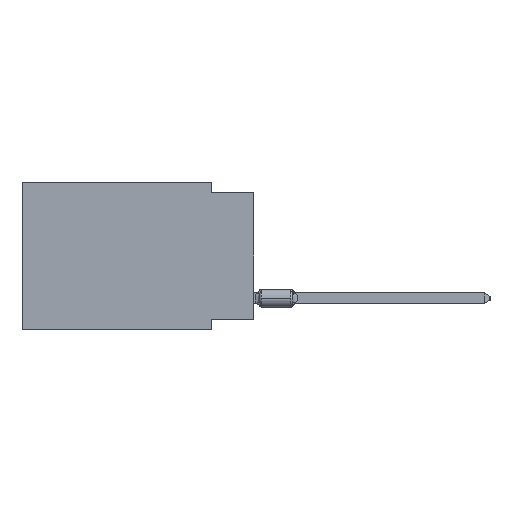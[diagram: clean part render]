
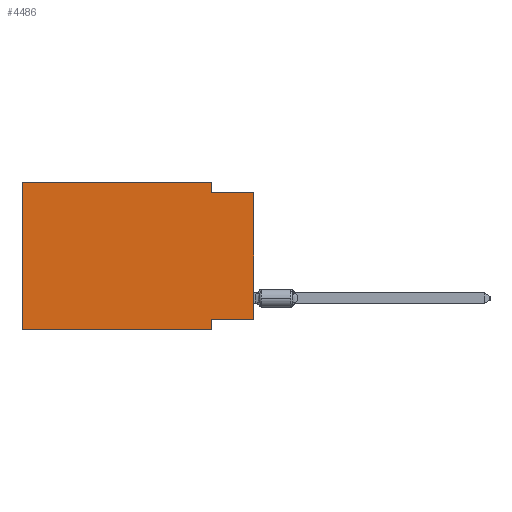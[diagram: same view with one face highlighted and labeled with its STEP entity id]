
A CAD part, left-side view. The second image highlights one B-rep face of the part: STEP entity #4486.
In plain terms, the highlighted planar face has unit normal (-1, 0, 0).
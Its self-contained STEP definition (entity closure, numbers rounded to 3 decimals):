
#250 = CARTESIAN_POINT ( 'NONE',  ( 0., 13.97, -8.89 ) ) ;
#287 = VERTEX_POINT ( 'NONE', #46574 ) ;
#1240 = EDGE_CURVE ( 'NONE', #6815, #39775, #16310, .T. ) ;
#1781 = EDGE_CURVE ( 'NONE', #7758, #39775, #43823, .T. ) ;
#1793 = EDGE_CURVE ( 'NONE', #24050, #10209, #14880, .T. ) ;
#2637 = VECTOR ( 'NONE', #41214, 1000. ) ;
#2808 = VERTEX_POINT ( 'NONE', #15003 ) ;
#3193 = DIRECTION ( 'NONE',  ( 0., 0., 1. ) ) ;
#3563 = CARTESIAN_POINT ( 'NONE',  ( 0., 2.54, -8.89 ) ) ;
#4158 = DIRECTION ( 'NONE',  ( 0., -1., 0. ) ) ;
#4486 = ADVANCED_FACE ( 'NONE', ( #8408 ), #12046, .F. ) ;
#5541 = AXIS2_PLACEMENT_3D ( 'NONE', #26904, #27388, #34438 ) ;
#5561 = CARTESIAN_POINT ( 'NONE',  ( 0., 13.97, -8.89 ) ) ;
#6062 = ORIENTED_EDGE ( 'NONE', *, *, #19565, .F. ) ;
#6815 = VERTEX_POINT ( 'NONE', #19381 ) ;
#7599 = LINE ( 'NONE', #34134, #39858 ) ;
#7758 = VERTEX_POINT ( 'NONE', #9679 ) ;
#7832 = VERTEX_POINT ( 'NONE', #5561 ) ;
#8134 = VECTOR ( 'NONE', #27026, 1000. ) ;
#8164 = CARTESIAN_POINT ( 'NONE',  ( 0., 2.54, 0. ) ) ;
#8408 = FACE_OUTER_BOUND ( 'NONE', #32817, .T. ) ;
#9679 = CARTESIAN_POINT ( 'NONE',  ( 0., 0., -8.255 ) ) ;
#10209 = VERTEX_POINT ( 'NONE', #8164 ) ;
#11531 = CARTESIAN_POINT ( 'NONE',  ( 0., 13.97, 0. ) ) ;
#11542 = CARTESIAN_POINT ( 'NONE',  ( 0., 13.97, 0. ) ) ;
#12046 = PLANE ( 'NONE',  #5541 ) ;
#12173 = CARTESIAN_POINT ( 'NONE',  ( 0., 0., -0.635 ) ) ;
#12879 = EDGE_CURVE ( 'NONE', #10209, #6815, #7599, .T. ) ;
#13235 = VECTOR ( 'NONE', #3193, 1000. ) ;
#13362 = EDGE_CURVE ( 'NONE', #7832, #2808, #33108, .T. ) ;
#14880 = LINE ( 'NONE', #41148, #31129 ) ;
#15003 = CARTESIAN_POINT ( 'NONE',  ( 0., 2.54, -8.89 ) ) ;
#15240 = LINE ( 'NONE', #23019, #30817 ) ;
#16310 = LINE ( 'NONE', #12173, #8134 ) ;
#16753 = ORIENTED_EDGE ( 'NONE', *, *, #1240, .F. ) ;
#18313 = DIRECTION ( 'NONE',  ( 0., 0., -1. ) ) ;
#18739 = ORIENTED_EDGE ( 'NONE', *, *, #13362, .T. ) ;
#19381 = CARTESIAN_POINT ( 'NONE',  ( 0., 2.54, -0.635 ) ) ;
#19565 = EDGE_CURVE ( 'NONE', #7758, #287, #15240, .T. ) ;
#22306 = DIRECTION ( 'NONE',  ( 0., 0., -1. ) ) ;
#22480 = LINE ( 'NONE', #11531, #2637 ) ;
#23019 = CARTESIAN_POINT ( 'NONE',  ( 0., 0., -8.255 ) ) ;
#24050 = VERTEX_POINT ( 'NONE', #11542 ) ;
#26904 = CARTESIAN_POINT ( 'NONE',  ( 0., 13.97, 0. ) ) ;
#27026 = DIRECTION ( 'NONE',  ( 0., -1., 0. ) ) ;
#27388 = DIRECTION ( 'NONE',  ( 1., 0., 0. ) ) ;
#29887 = ORIENTED_EDGE ( 'NONE', *, *, #35350, .F. ) ;
#30703 = VECTOR ( 'NONE', #22306, 1000. ) ;
#30817 = VECTOR ( 'NONE', #41501, 1000. ) ;
#31129 = VECTOR ( 'NONE', #4158, 1000. ) ;
#32084 = ORIENTED_EDGE ( 'NONE', *, *, #12879, .F. ) ;
#32817 = EDGE_LOOP ( 'NONE', ( #39248, #16753, #32084, #45285, #29887, #18739, #46748, #6062 ) ) ;
#33108 = LINE ( 'NONE', #250, #39134 ) ;
#33596 = DIRECTION ( 'NONE',  ( 0., -1., 0. ) ) ;
#34134 = CARTESIAN_POINT ( 'NONE',  ( 0., 2.54, 0. ) ) ;
#34438 = DIRECTION ( 'NONE',  ( 0., 0., -1. ) ) ;
#35350 = EDGE_CURVE ( 'NONE', #7832, #24050, #22480, .T. ) ;
#36129 = EDGE_CURVE ( 'NONE', #287, #2808, #36914, .T. ) ;
#36544 = CARTESIAN_POINT ( 'NONE',  ( 0., 0., -0.635 ) ) ;
#36914 = LINE ( 'NONE', #3563, #30703 ) ;
#39134 = VECTOR ( 'NONE', #33596, 1000. ) ;
#39248 = ORIENTED_EDGE ( 'NONE', *, *, #1781, .T. ) ;
#39775 = VERTEX_POINT ( 'NONE', #36544 ) ;
#39858 = VECTOR ( 'NONE', #18313, 1000. ) ;
#40184 = CARTESIAN_POINT ( 'NONE',  ( 0., 0., 0. ) ) ;
#41148 = CARTESIAN_POINT ( 'NONE',  ( 0., 13.97, 0. ) ) ;
#41214 = DIRECTION ( 'NONE',  ( 0., 0., 1. ) ) ;
#41501 = DIRECTION ( 'NONE',  ( 0., 1., 0. ) ) ;
#43823 = LINE ( 'NONE', #40184, #13235 ) ;
#45285 = ORIENTED_EDGE ( 'NONE', *, *, #1793, .F. ) ;
#46574 = CARTESIAN_POINT ( 'NONE',  ( 0., 2.54, -8.255 ) ) ;
#46748 = ORIENTED_EDGE ( 'NONE', *, *, #36129, .F. ) ;
